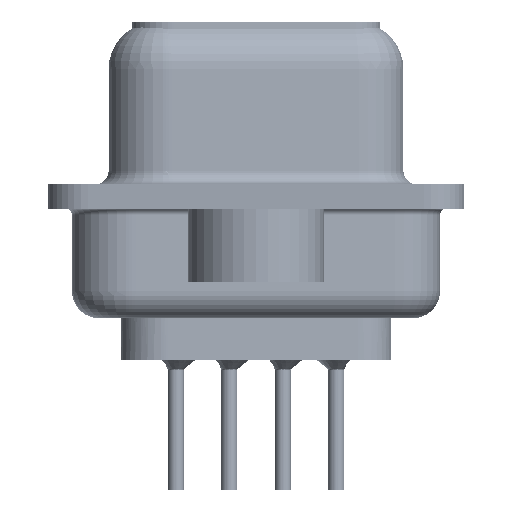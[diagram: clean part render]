
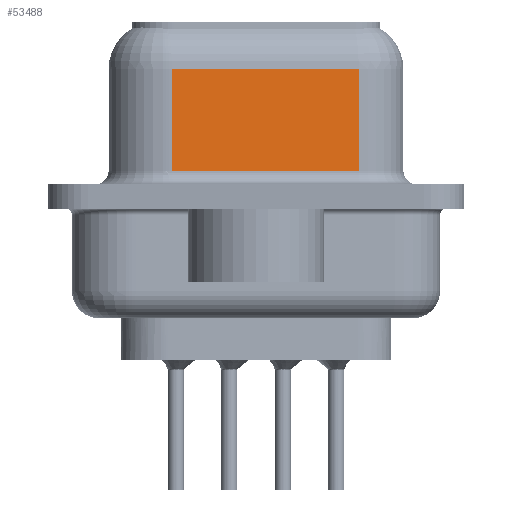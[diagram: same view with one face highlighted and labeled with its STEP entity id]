
A CAD part, left-side view. The second image highlights one B-rep face of the part: STEP entity #53488.
In plain terms, the highlighted planar face has unit normal (-0.985, -0.174, 0).
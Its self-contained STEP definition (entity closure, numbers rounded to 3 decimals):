
#2283 = EDGE_LOOP ( 'NONE', ( #38224, #12482, #13729, #25462 ) ) ;
#2342 = LINE ( 'NONE', #25474, #51858 ) ;
#2477 = DIRECTION ( 'NONE',  ( 0.174, -0.985, 0. ) ) ;
#4945 = DIRECTION ( 'NONE',  ( -0.174, 0.985, 0. ) ) ;
#5560 = VECTOR ( 'NONE', #4945, 1000. ) ;
#8534 = VERTEX_POINT ( 'NONE', #17327 ) ;
#10994 = CARTESIAN_POINT ( 'NONE',  ( 5.697, -3.797, 0.95 ) ) ;
#12482 = ORIENTED_EDGE ( 'NONE', *, *, #31871, .T. ) ;
#13729 = ORIENTED_EDGE ( 'NONE', *, *, #44728, .T. ) ;
#16923 = CARTESIAN_POINT ( 'NONE',  ( 4.48, 3.103, 6.45 ) ) ;
#17327 = CARTESIAN_POINT ( 'NONE',  ( 5.697, -3.797, 0.95 ) ) ;
#18700 = VECTOR ( 'NONE', #2477, 1000. ) ;
#19062 = VERTEX_POINT ( 'NONE', #36696 ) ;
#19121 = CARTESIAN_POINT ( 'NONE',  ( 5.697, -3.797, 6.45 ) ) ;
#21836 = PLANE ( 'NONE',  #44389 ) ;
#25462 = ORIENTED_EDGE ( 'NONE', *, *, #39131, .T. ) ;
#25474 = CARTESIAN_POINT ( 'NONE',  ( 5.697, -3.797, 6.45 ) ) ;
#26906 = VERTEX_POINT ( 'NONE', #35335 ) ;
#30643 = FACE_OUTER_BOUND ( 'NONE', #2283, .T. ) ;
#31632 = LINE ( 'NONE', #45125, #5560 ) ;
#31735 = CARTESIAN_POINT ( 'NONE',  ( 5.697, -3.797, 4.7 ) ) ;
#31871 = EDGE_CURVE ( 'NONE', #48202, #19062, #31632, .T. ) ;
#35335 = CARTESIAN_POINT ( 'NONE',  ( 4.48, 3.103, 0.95 ) ) ;
#36696 = CARTESIAN_POINT ( 'NONE',  ( 4.48, 3.103, 4.7 ) ) ;
#38224 = ORIENTED_EDGE ( 'NONE', *, *, #54792, .F. ) ;
#39131 = EDGE_CURVE ( 'NONE', #26906, #8534, #56384, .T. ) ;
#40642 = LINE ( 'NONE', #16923, #52748 ) ;
#44389 = AXIS2_PLACEMENT_3D ( 'NONE', #19121, #50191, #54289 ) ;
#44728 = EDGE_CURVE ( 'NONE', #19062, #26906, #40642, .T. ) ;
#45125 = CARTESIAN_POINT ( 'NONE',  ( 5.697, -3.797, 4.7 ) ) ;
#48202 = VERTEX_POINT ( 'NONE', #31735 ) ;
#50191 = DIRECTION ( 'NONE',  ( 0.985, 0.174, 0. ) ) ;
#51858 = VECTOR ( 'NONE', #55684, 1000. ) ;
#52659 = DIRECTION ( 'NONE',  ( 0., 0., -1. ) ) ;
#52748 = VECTOR ( 'NONE', #52659, 1000. ) ;
#53488 = ADVANCED_FACE ( 'NONE', ( #30643 ), #21836, .F. ) ;
#54289 = DIRECTION ( 'NONE',  ( -0.174, 0.985, 0. ) ) ;
#54792 = EDGE_CURVE ( 'NONE', #48202, #8534, #2342, .T. ) ;
#55684 = DIRECTION ( 'NONE',  ( 0., 0., -1. ) ) ;
#56384 = LINE ( 'NONE', #10994, #18700 ) ;
